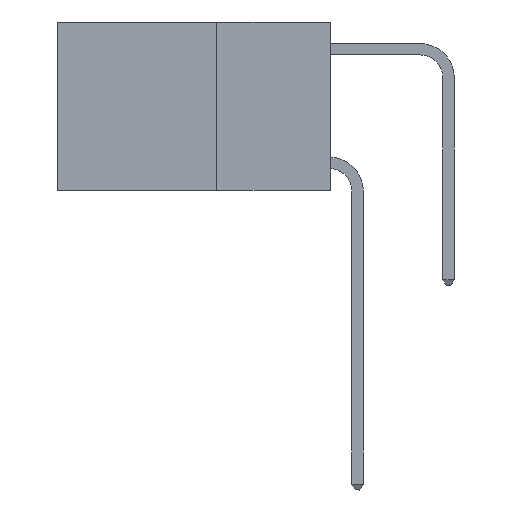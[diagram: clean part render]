
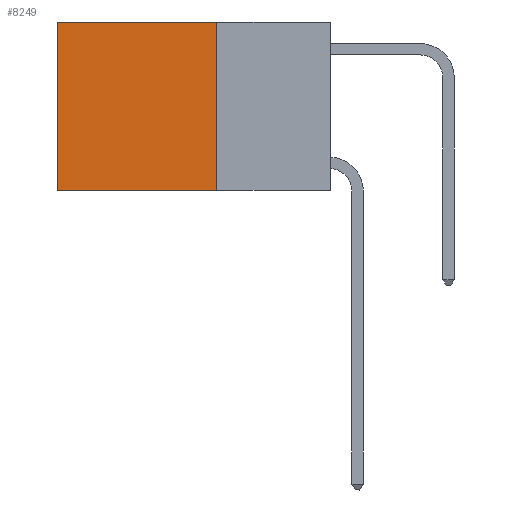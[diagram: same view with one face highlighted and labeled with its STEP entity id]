
A CAD part, left-side view. The second image highlights one B-rep face of the part: STEP entity #8249.
In plain terms, the highlighted planar face has unit normal (-1, 0, 0).
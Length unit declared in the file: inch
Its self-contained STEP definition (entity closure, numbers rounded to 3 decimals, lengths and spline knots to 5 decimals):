
#1594 = CARTESIAN_POINT ( 'NONE',  ( 0.2625, 0.25, 0. ) ) ;
#1715 = DIRECTION ( 'NONE',  ( 1., 0., 0. ) ) ;
#1802 = LINE ( 'NONE', #15900, #8459 ) ;
#2028 = DIRECTION ( 'NONE',  ( 0., 1., 0. ) ) ;
#2056 = EDGE_LOOP ( 'NONE', ( #7130, #8061, #3016, #7632 ) ) ;
#2209 = DIRECTION ( 'NONE',  ( 0., 0., -1. ) ) ;
#2528 = VERTEX_POINT ( 'NONE', #10727 ) ;
#2920 = PLANE ( 'NONE',  #8262 ) ;
#3016 = ORIENTED_EDGE ( 'NONE', *, *, #7058, .F. ) ;
#5413 = LINE ( 'NONE', #17149, #17097 ) ;
#7058 = EDGE_CURVE ( 'NONE', #16973, #7778, #1802, .T. ) ;
#7130 = ORIENTED_EDGE ( 'NONE', *, *, #14111, .T. ) ;
#7304 = CARTESIAN_POINT ( 'NONE',  ( 0.2625, 0.25, -0.37 ) ) ;
#7349 = EDGE_CURVE ( 'NONE', #16973, #8443, #13053, .T. ) ;
#7601 = VECTOR ( 'NONE', #2028, 39.37008 ) ;
#7632 = ORIENTED_EDGE ( 'NONE', *, *, #7349, .T. ) ;
#7778 = VERTEX_POINT ( 'NONE', #15024 ) ;
#7858 = CARTESIAN_POINT ( 'NONE',  ( 0.2625, 0.25, 0. ) ) ;
#8061 = ORIENTED_EDGE ( 'NONE', *, *, #8912, .F. ) ;
#8249 = ADVANCED_FACE ( 'NONE', ( #14264 ), #2920, .F. ) ;
#8262 = AXIS2_PLACEMENT_3D ( 'NONE', #1594, #1715, #16290 ) ;
#8443 = VERTEX_POINT ( 'NONE', #8684 ) ;
#8459 = VECTOR ( 'NONE', #13399, 39.37008 ) ;
#8684 = CARTESIAN_POINT ( 'NONE',  ( 0.2625, 0.6, 0. ) ) ;
#8912 = EDGE_CURVE ( 'NONE', #7778, #2528, #11175, .T. ) ;
#10727 = CARTESIAN_POINT ( 'NONE',  ( 0.2625, 0.6, -0.37 ) ) ;
#11175 = LINE ( 'NONE', #7304, #7601 ) ;
#12806 = DIRECTION ( 'NONE',  ( 0., 1., 0. ) ) ;
#12837 = VECTOR ( 'NONE', #12806, 39.37008 ) ;
#13053 = LINE ( 'NONE', #15379, #12837 ) ;
#13399 = DIRECTION ( 'NONE',  ( 0., 0., -1. ) ) ;
#14111 = EDGE_CURVE ( 'NONE', #8443, #2528, #5413, .T. ) ;
#14264 = FACE_OUTER_BOUND ( 'NONE', #2056, .T. ) ;
#15024 = CARTESIAN_POINT ( 'NONE',  ( 0.2625, 0.25, -0.37 ) ) ;
#15379 = CARTESIAN_POINT ( 'NONE',  ( 0.2625, 0.25, 0. ) ) ;
#15900 = CARTESIAN_POINT ( 'NONE',  ( 0.2625, 0.25, 0. ) ) ;
#16290 = DIRECTION ( 'NONE',  ( 0., 0., -1. ) ) ;
#16973 = VERTEX_POINT ( 'NONE', #7858 ) ;
#17097 = VECTOR ( 'NONE', #2209, 39.37008 ) ;
#17149 = CARTESIAN_POINT ( 'NONE',  ( 0.2625, 0.6, 0. ) ) ;
